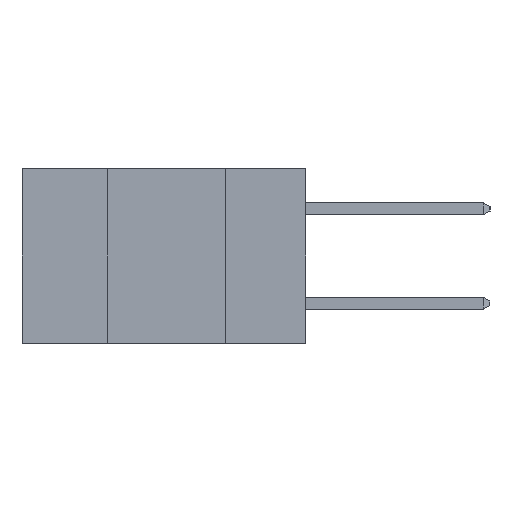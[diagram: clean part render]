
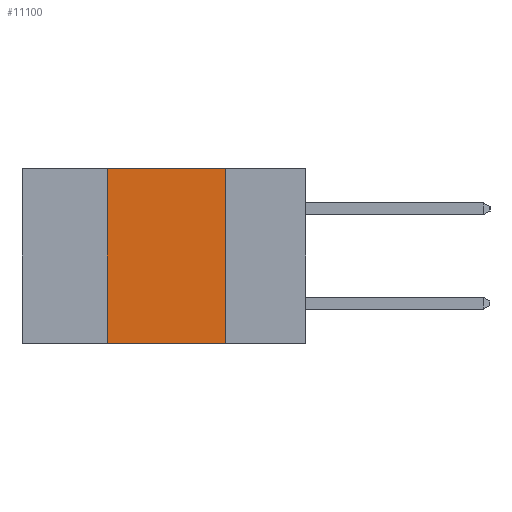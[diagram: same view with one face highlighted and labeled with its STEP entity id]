
A CAD part, left-side view. The second image highlights one B-rep face of the part: STEP entity #11100.
In plain terms, the highlighted planar face has unit normal (-1, 0, 0).
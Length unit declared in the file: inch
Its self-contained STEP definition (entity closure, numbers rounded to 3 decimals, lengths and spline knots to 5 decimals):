
#98 = EDGE_LOOP ( 'NONE', ( #7284, #12952, #9817, #1681 ) ) ;
#1062 = VERTEX_POINT ( 'NONE', #21909 ) ;
#1113 = VERTEX_POINT ( 'NONE', #7363 ) ;
#1681 = ORIENTED_EDGE ( 'NONE', *, *, #5432, .T. ) ;
#2831 = CARTESIAN_POINT ( 'NONE',  ( 0., 0.6, -0.37 ) ) ;
#3229 = AXIS2_PLACEMENT_3D ( 'NONE', #5066, #23348, #12461 ) ;
#4239 = CARTESIAN_POINT ( 'NONE',  ( 0., 0.42, -0.37 ) ) ;
#4423 = LINE ( 'NONE', #2831, #13054 ) ;
#5066 = CARTESIAN_POINT ( 'NONE',  ( 0., 0.6, 0. ) ) ;
#5432 = EDGE_CURVE ( 'NONE', #10364, #1062, #4423, .T. ) ;
#5849 = VECTOR ( 'NONE', #15241, 39.37008 ) ;
#6367 = CARTESIAN_POINT ( 'NONE',  ( 0., 0.17, 0. ) ) ;
#6662 = EDGE_CURVE ( 'NONE', #10364, #1113, #15611, .T. ) ;
#7284 = ORIENTED_EDGE ( 'NONE', *, *, #10328, .F. ) ;
#7363 = CARTESIAN_POINT ( 'NONE',  ( 0., 0.42, 0. ) ) ;
#7767 = LINE ( 'NONE', #16075, #21781 ) ;
#7878 = EDGE_CURVE ( 'NONE', #1113, #10899, #7767, .T. ) ;
#9408 = LINE ( 'NONE', #14092, #22821 ) ;
#9817 = ORIENTED_EDGE ( 'NONE', *, *, #6662, .F. ) ;
#10328 = EDGE_CURVE ( 'NONE', #10899, #1062, #9408, .T. ) ;
#10364 = VERTEX_POINT ( 'NONE', #12323 ) ;
#10899 = VERTEX_POINT ( 'NONE', #6367 ) ;
#11100 = ADVANCED_FACE ( 'NONE', ( #16574 ), #19743, .F. ) ;
#11988 = DIRECTION ( 'NONE',  ( 0., -1., 0. ) ) ;
#12323 = CARTESIAN_POINT ( 'NONE',  ( 0., 0.42, -0.37 ) ) ;
#12461 = DIRECTION ( 'NONE',  ( 0., 0., -1. ) ) ;
#12952 = ORIENTED_EDGE ( 'NONE', *, *, #7878, .F. ) ;
#13054 = VECTOR ( 'NONE', #11988, 39.37008 ) ;
#14092 = CARTESIAN_POINT ( 'NONE',  ( 0., 0.17, -0.37 ) ) ;
#15241 = DIRECTION ( 'NONE',  ( 0., 0., 1. ) ) ;
#15611 = LINE ( 'NONE', #4239, #5849 ) ;
#15942 = DIRECTION ( 'NONE',  ( 0., 0., -1. ) ) ;
#16075 = CARTESIAN_POINT ( 'NONE',  ( 0., 0.6, 0. ) ) ;
#16574 = FACE_OUTER_BOUND ( 'NONE', #98, .T. ) ;
#17908 = DIRECTION ( 'NONE',  ( 0., -1., 0. ) ) ;
#19743 = PLANE ( 'NONE',  #3229 ) ;
#21781 = VECTOR ( 'NONE', #17908, 39.37008 ) ;
#21909 = CARTESIAN_POINT ( 'NONE',  ( 0., 0.17, -0.37 ) ) ;
#22821 = VECTOR ( 'NONE', #15942, 39.37008 ) ;
#23348 = DIRECTION ( 'NONE',  ( 1., 0., 0. ) ) ;
